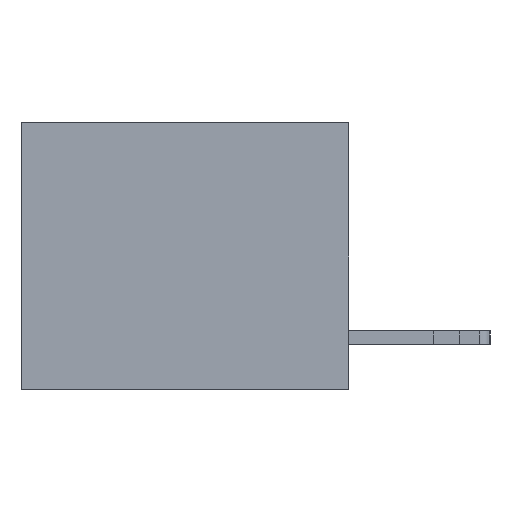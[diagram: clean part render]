
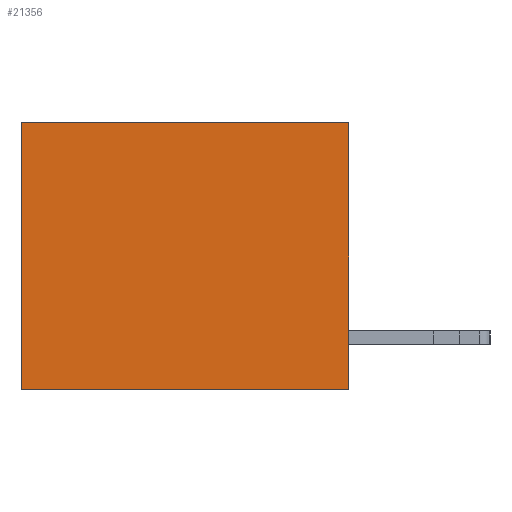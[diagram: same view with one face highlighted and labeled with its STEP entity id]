
A CAD part, left-side view. The second image highlights one B-rep face of the part: STEP entity #21356.
In plain terms, the highlighted planar face has unit normal (-1, 0, 0).
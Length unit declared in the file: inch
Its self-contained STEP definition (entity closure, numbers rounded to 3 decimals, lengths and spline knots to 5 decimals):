
#3291 = DIRECTION ( 'NONE',  ( 0., 0., -1. ) ) ;
#3338 = DIRECTION ( 'NONE',  ( 0., 1., 0. ) ) ;
#3760 = LINE ( 'NONE', #5702, #28786 ) ;
#5219 = VERTEX_POINT ( 'NONE', #27751 ) ;
#5702 = CARTESIAN_POINT ( 'NONE',  ( 0.3165, 0.6, -0.49 ) ) ;
#5889 = VERTEX_POINT ( 'NONE', #18264 ) ;
#6531 = CARTESIAN_POINT ( 'NONE',  ( 0.3165, 0., 0. ) ) ;
#7063 = VERTEX_POINT ( 'NONE', #6531 ) ;
#7361 = CARTESIAN_POINT ( 'NONE',  ( 0.3165, 0., -0.49 ) ) ;
#7984 = ORIENTED_EDGE ( 'NONE', *, *, #26397, .F. ) ;
#8755 = CARTESIAN_POINT ( 'NONE',  ( 0.3165, 0., -0.49 ) ) ;
#9848 = EDGE_CURVE ( 'NONE', #7063, #5889, #24416, .T. ) ;
#10052 = EDGE_LOOP ( 'NONE', ( #12076, #7984, #27463, #20035 ) ) ;
#10077 = VERTEX_POINT ( 'NONE', #27520 ) ;
#10759 = AXIS2_PLACEMENT_3D ( 'NONE', #7361, #19296, #14665 ) ;
#11737 = PLANE ( 'NONE',  #10759 ) ;
#12076 = ORIENTED_EDGE ( 'NONE', *, *, #27095, .T. ) ;
#12613 = DIRECTION ( 'NONE',  ( 0., 0., -1. ) ) ;
#12665 = FACE_OUTER_BOUND ( 'NONE', #10052, .T. ) ;
#13615 = VECTOR ( 'NONE', #3338, 39.37008 ) ;
#14665 = DIRECTION ( 'NONE',  ( 0., 0., -1. ) ) ;
#16733 = EDGE_CURVE ( 'NONE', #7063, #10077, #25178, .T. ) ;
#16905 = CARTESIAN_POINT ( 'NONE',  ( 0.3165, 0., 0. ) ) ;
#18264 = CARTESIAN_POINT ( 'NONE',  ( 0.3165, 0.6, 0. ) ) ;
#19296 = DIRECTION ( 'NONE',  ( 1., 0., 0. ) ) ;
#19759 = CARTESIAN_POINT ( 'NONE',  ( 0.3165, 0., -0.49 ) ) ;
#20035 = ORIENTED_EDGE ( 'NONE', *, *, #9848, .T. ) ;
#21356 = ADVANCED_FACE ( 'NONE', ( #12665 ), #11737, .F. ) ;
#23598 = DIRECTION ( 'NONE',  ( 0., 1., 0. ) ) ;
#24416 = LINE ( 'NONE', #16905, #28782 ) ;
#25178 = LINE ( 'NONE', #19759, #27716 ) ;
#26397 = EDGE_CURVE ( 'NONE', #10077, #5219, #26695, .T. ) ;
#26695 = LINE ( 'NONE', #8755, #13615 ) ;
#27095 = EDGE_CURVE ( 'NONE', #5889, #5219, #3760, .T. ) ;
#27463 = ORIENTED_EDGE ( 'NONE', *, *, #16733, .F. ) ;
#27520 = CARTESIAN_POINT ( 'NONE',  ( 0.3165, 0., -0.49 ) ) ;
#27716 = VECTOR ( 'NONE', #12613, 39.37008 ) ;
#27751 = CARTESIAN_POINT ( 'NONE',  ( 0.3165, 0.6, -0.49 ) ) ;
#28782 = VECTOR ( 'NONE', #23598, 39.37008 ) ;
#28786 = VECTOR ( 'NONE', #3291, 39.37008 ) ;
